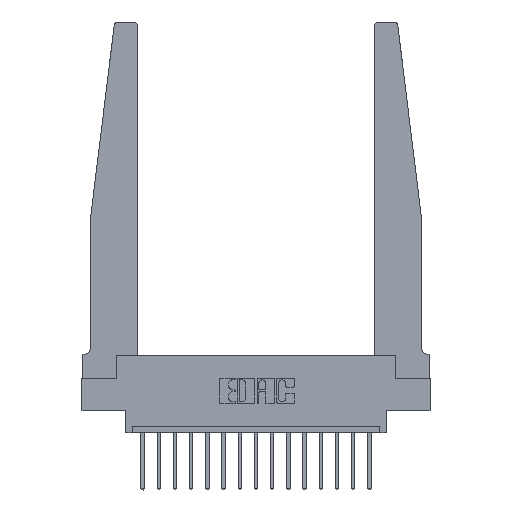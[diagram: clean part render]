
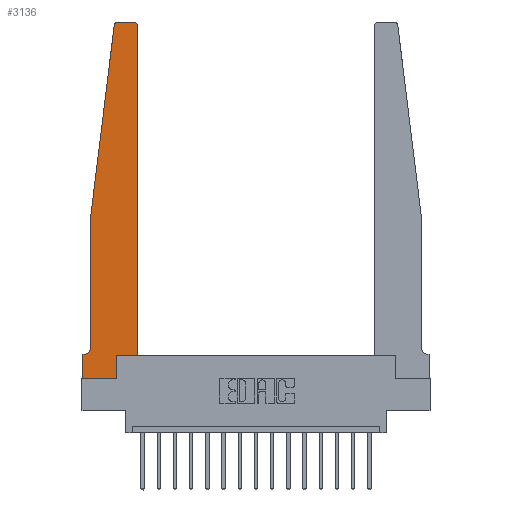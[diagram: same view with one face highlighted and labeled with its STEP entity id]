
A CAD part, top view. The second image highlights one B-rep face of the part: STEP entity #3136.
In plain terms, the highlighted planar face has unit normal (0, 0, 1).
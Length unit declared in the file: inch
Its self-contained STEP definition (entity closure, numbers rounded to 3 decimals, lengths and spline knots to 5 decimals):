
#24 = CARTESIAN_POINT ( 'NONE',  ( 0.2605, 0.18, 0.37 ) ) ;
#217 = VECTOR ( 'NONE', #6823, 39.37008 ) ;
#565 = EDGE_CURVE ( 'NONE', #17784, #1120, #4907, .T. ) ;
#603 = CARTESIAN_POINT ( 'NONE',  ( 0.2605, 0.18, 0.37 ) ) ;
#739 = CARTESIAN_POINT ( 'NONE',  ( 0.2605, 0., 0.37 ) ) ;
#753 = EDGE_CURVE ( 'NONE', #17053, #9344, #16171, .T. ) ;
#767 = EDGE_CURVE ( 'NONE', #6383, #14411, #16601, .T. ) ;
#781 = VERTEX_POINT ( 'NONE', #24 ) ;
#783 = CARTESIAN_POINT ( 'NONE',  ( 0., 0.1875, 0.37 ) ) ;
#1115 = DIRECTION ( 'NONE',  ( 1., 0., 0. ) ) ;
#1120 = VERTEX_POINT ( 'NONE', #10932 ) ;
#1281 = EDGE_CURVE ( 'NONE', #17518, #17784, #7075, .T. ) ;
#1398 = ORIENTED_EDGE ( 'NONE', *, *, #4005, .T. ) ;
#1404 = CARTESIAN_POINT ( 'NONE',  ( 0.395, 2.72, 0.37 ) ) ;
#1419 = CIRCLE ( 'NONE', #3307, 0.05 ) ;
#1535 = VERTEX_POINT ( 'NONE', #1721 ) ;
#1721 = CARTESIAN_POINT ( 'NONE',  ( 0.065, 0.2375, 0.37 ) ) ;
#1876 = CARTESIAN_POINT ( 'NONE',  ( 0.015, 0.1875, 0.37 ) ) ;
#1967 = AXIS2_PLACEMENT_3D ( 'NONE', #17026, #11538, #12882 ) ;
#2165 = DIRECTION ( 'NONE',  ( 0., -1., 0. ) ) ;
#2670 = DIRECTION ( 'NONE',  ( 1., 0., 0. ) ) ;
#2794 = DIRECTION ( 'NONE',  ( 0., 0., 1. ) ) ;
#2974 = LINE ( 'NONE', #17825, #17217 ) ;
#2985 = DIRECTION ( 'NONE',  ( 1., 0., 0. ) ) ;
#3136 = ADVANCED_FACE ( 'NONE', ( #11517 ), #10154, .T. ) ;
#3225 = LINE ( 'NONE', #603, #15996 ) ;
#3307 = AXIS2_PLACEMENT_3D ( 'NONE', #5930, #6471, #9275 ) ;
#3366 = CARTESIAN_POINT ( 'NONE',  ( 0.065, 1.25, 0.37 ) ) ;
#3775 = CARTESIAN_POINT ( 'NONE',  ( 0., 0., 0.37 ) ) ;
#4001 = CARTESIAN_POINT ( 'NONE',  ( 0.25, 2.75, 0.37 ) ) ;
#4005 = EDGE_CURVE ( 'NONE', #9344, #13662, #12588, .T. ) ;
#4214 = CARTESIAN_POINT ( 'NONE',  ( 0.065, 0.1875, 0.37 ) ) ;
#4446 = LINE ( 'NONE', #15366, #9011 ) ;
#4590 = AXIS2_PLACEMENT_3D ( 'NONE', #10977, #9559, #1115 ) ;
#4801 = EDGE_CURVE ( 'NONE', #11404, #781, #3225, .T. ) ;
#4907 = LINE ( 'NONE', #16420, #217 ) ;
#4960 = ORIENTED_EDGE ( 'NONE', *, *, #6781, .T. ) ;
#5260 = VERTEX_POINT ( 'NONE', #15350 ) ;
#5499 = ORIENTED_EDGE ( 'NONE', *, *, #6174, .T. ) ;
#5655 = ORIENTED_EDGE ( 'NONE', *, *, #6503, .T. ) ;
#5759 = ORIENTED_EDGE ( 'NONE', *, *, #12717, .T. ) ;
#5767 = VECTOR ( 'NONE', #2165, 39.37008 ) ;
#5930 = CARTESIAN_POINT ( 'NONE',  ( 0.015, 0.2375, 0.37 ) ) ;
#6174 = EDGE_CURVE ( 'NONE', #14411, #17518, #12703, .T. ) ;
#6383 = VERTEX_POINT ( 'NONE', #11716 ) ;
#6471 = DIRECTION ( 'NONE',  ( 0., 0., -1. ) ) ;
#6503 = EDGE_CURVE ( 'NONE', #781, #5260, #15503, .T. ) ;
#6727 = DIRECTION ( 'NONE',  ( 0., 1., 0. ) ) ;
#6781 = EDGE_CURVE ( 'NONE', #1120, #1535, #9489, .T. ) ;
#6823 = DIRECTION ( 'NONE',  ( -0.122, -0.992, 0. ) ) ;
#7013 = DIRECTION ( 'NONE',  ( -1., 0., 0. ) ) ;
#7075 = CIRCLE ( 'NONE', #4590, 0.03 ) ;
#7646 = CARTESIAN_POINT ( 'NONE',  ( 0.24675, 2.72367, 0.37 ) ) ;
#7715 = ORIENTED_EDGE ( 'NONE', *, *, #753, .T. ) ;
#7812 = DIRECTION ( 'NONE',  ( 1., 0., 0. ) ) ;
#7890 = CARTESIAN_POINT ( 'NONE',  ( 0.425, 0.18, 0.37 ) ) ;
#8256 = DIRECTION ( 'NONE',  ( 0., -1., 0. ) ) ;
#9011 = VECTOR ( 'NONE', #2985, 39.37008 ) ;
#9098 = ORIENTED_EDGE ( 'NONE', *, *, #16840, .T. ) ;
#9275 = DIRECTION ( 'NONE',  ( -1., 0., 0. ) ) ;
#9341 = DIRECTION ( 'NONE',  ( -1., 0., 0. ) ) ;
#9344 = VERTEX_POINT ( 'NONE', #783 ) ;
#9406 = ORIENTED_EDGE ( 'NONE', *, *, #13987, .T. ) ;
#9489 = LINE ( 'NONE', #3366, #5767 ) ;
#9559 = DIRECTION ( 'NONE',  ( 0., 0., 1. ) ) ;
#9744 = AXIS2_PLACEMENT_3D ( 'NONE', #1404, #2794, #2670 ) ;
#9862 = CARTESIAN_POINT ( 'NONE',  ( 0.27653, 2.75, 0.37 ) ) ;
#10154 = PLANE ( 'NONE',  #1967 ) ;
#10393 = CARTESIAN_POINT ( 'NONE',  ( 0., 0., 0.37 ) ) ;
#10932 = CARTESIAN_POINT ( 'NONE',  ( 0.065, 1.25, 0.37 ) ) ;
#10977 = CARTESIAN_POINT ( 'NONE',  ( 0.27653, 2.72, 0.37 ) ) ;
#11404 = VERTEX_POINT ( 'NONE', #739 ) ;
#11517 = FACE_OUTER_BOUND ( 'NONE', #16707, .T. ) ;
#11538 = DIRECTION ( 'NONE',  ( 0., 0., 1. ) ) ;
#11716 = CARTESIAN_POINT ( 'NONE',  ( 0.425, 2.72, 0.37 ) ) ;
#11825 = VECTOR ( 'NONE', #9341, 39.37008 ) ;
#12041 = ORIENTED_EDGE ( 'NONE', *, *, #565, .T. ) ;
#12588 = LINE ( 'NONE', #3775, #13676 ) ;
#12597 = ORIENTED_EDGE ( 'NONE', *, *, #1281, .T. ) ;
#12703 = LINE ( 'NONE', #4001, #11825 ) ;
#12717 = EDGE_CURVE ( 'NONE', #5260, #6383, #2974, .T. ) ;
#12789 = ORIENTED_EDGE ( 'NONE', *, *, #767, .T. ) ;
#12882 = DIRECTION ( 'NONE',  ( 1., 0., 0. ) ) ;
#13418 = ORIENTED_EDGE ( 'NONE', *, *, #4801, .T. ) ;
#13662 = VERTEX_POINT ( 'NONE', #10393 ) ;
#13676 = VECTOR ( 'NONE', #8256, 39.37008 ) ;
#13987 = EDGE_CURVE ( 'NONE', #13662, #11404, #4446, .T. ) ;
#14411 = VERTEX_POINT ( 'NONE', #16830 ) ;
#15350 = CARTESIAN_POINT ( 'NONE',  ( 0.425, 0.18, 0.37 ) ) ;
#15366 = CARTESIAN_POINT ( 'NONE',  ( 0., 0., 0.37 ) ) ;
#15503 = LINE ( 'NONE', #7890, #16591 ) ;
#15994 = DIRECTION ( 'NONE',  ( 0., 1., 0. ) ) ;
#15996 = VECTOR ( 'NONE', #15994, 39.37008 ) ;
#16171 = LINE ( 'NONE', #4214, #17674 ) ;
#16420 = CARTESIAN_POINT ( 'NONE',  ( 0.065, 1.25, 0.37 ) ) ;
#16591 = VECTOR ( 'NONE', #7812, 39.37008 ) ;
#16601 = CIRCLE ( 'NONE', #9744, 0.03 ) ;
#16707 = EDGE_LOOP ( 'NONE', ( #5499, #12597, #12041, #4960, #9098, #7715, #1398, #9406, #13418, #5655, #5759, #12789 ) ) ;
#16830 = CARTESIAN_POINT ( 'NONE',  ( 0.395, 2.75, 0.37 ) ) ;
#16840 = EDGE_CURVE ( 'NONE', #1535, #17053, #1419, .T. ) ;
#17026 = CARTESIAN_POINT ( 'NONE',  ( 0., 0.1875, 0.37 ) ) ;
#17053 = VERTEX_POINT ( 'NONE', #1876 ) ;
#17217 = VECTOR ( 'NONE', #6727, 39.37008 ) ;
#17518 = VERTEX_POINT ( 'NONE', #9862 ) ;
#17674 = VECTOR ( 'NONE', #7013, 39.37008 ) ;
#17784 = VERTEX_POINT ( 'NONE', #7646 ) ;
#17825 = CARTESIAN_POINT ( 'NONE',  ( 0.425, 0.18, 0.37 ) ) ;
